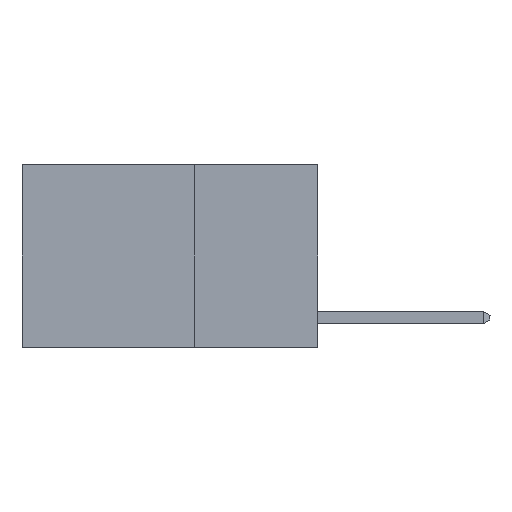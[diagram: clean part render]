
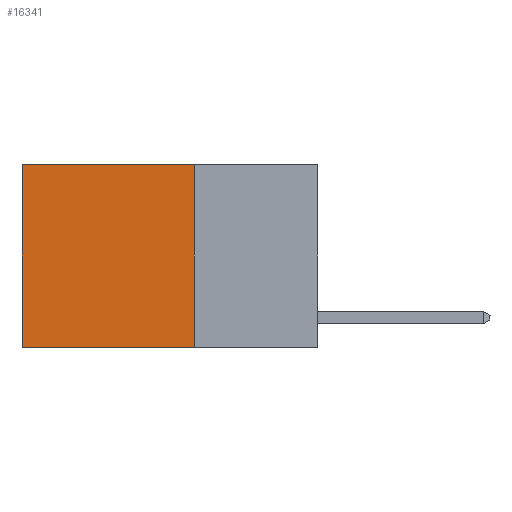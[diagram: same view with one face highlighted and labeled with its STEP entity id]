
A CAD part, left-side view. The second image highlights one B-rep face of the part: STEP entity #16341.
In plain terms, the highlighted planar face has unit normal (-1, 0, 0).
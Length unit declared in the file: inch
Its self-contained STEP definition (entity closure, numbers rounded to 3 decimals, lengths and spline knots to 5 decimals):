
#420 = CARTESIAN_POINT ( 'NONE',  ( 0.2625, 0.25, 0. ) ) ;
#433 = LINE ( 'NONE', #10669, #5865 ) ;
#895 = CARTESIAN_POINT ( 'NONE',  ( 0.2625, 0.25, 0. ) ) ;
#1762 = PLANE ( 'NONE',  #6375 ) ;
#1812 = ORIENTED_EDGE ( 'NONE', *, *, #13394, .F. ) ;
#3799 = EDGE_CURVE ( 'NONE', #4069, #9972, #10710, .T. ) ;
#4069 = VERTEX_POINT ( 'NONE', #8999 ) ;
#4175 = VERTEX_POINT ( 'NONE', #895 ) ;
#4338 = FACE_OUTER_BOUND ( 'NONE', #16299, .T. ) ;
#4739 = DIRECTION ( 'NONE',  ( 0., 1., 0. ) ) ;
#5096 = DIRECTION ( 'NONE',  ( 0., 0., -1. ) ) ;
#5238 = DIRECTION ( 'NONE',  ( 0., 0., -1. ) ) ;
#5668 = VECTOR ( 'NONE', #5238, 39.37008 ) ;
#5865 = VECTOR ( 'NONE', #5096, 39.37008 ) ;
#6375 = AXIS2_PLACEMENT_3D ( 'NONE', #420, #12952, #7456 ) ;
#7456 = DIRECTION ( 'NONE',  ( 0., 0., -1. ) ) ;
#8883 = CARTESIAN_POINT ( 'NONE',  ( 0.2625, 0.6, -0.37 ) ) ;
#8999 = CARTESIAN_POINT ( 'NONE',  ( 0.2625, 0.6, 0. ) ) ;
#9010 = CARTESIAN_POINT ( 'NONE',  ( 0.2625, 0.25, -0.37 ) ) ;
#9330 = LINE ( 'NONE', #15274, #12455 ) ;
#9401 = CARTESIAN_POINT ( 'NONE',  ( 0.2625, 0.25, -0.37 ) ) ;
#9972 = VERTEX_POINT ( 'NONE', #8883 ) ;
#10669 = CARTESIAN_POINT ( 'NONE',  ( 0.2625, 0.25, 0. ) ) ;
#10710 = LINE ( 'NONE', #10927, #5668 ) ;
#10927 = CARTESIAN_POINT ( 'NONE',  ( 0.2625, 0.6, 0. ) ) ;
#11186 = ORIENTED_EDGE ( 'NONE', *, *, #3799, .T. ) ;
#11480 = ORIENTED_EDGE ( 'NONE', *, *, #14968, .F. ) ;
#12455 = VECTOR ( 'NONE', #15452, 39.37008 ) ;
#12503 = VECTOR ( 'NONE', #4739, 39.37008 ) ;
#12833 = VERTEX_POINT ( 'NONE', #9401 ) ;
#12952 = DIRECTION ( 'NONE',  ( 1., 0., 0. ) ) ;
#13394 = EDGE_CURVE ( 'NONE', #4175, #12833, #433, .T. ) ;
#14114 = EDGE_CURVE ( 'NONE', #4175, #4069, #9330, .T. ) ;
#14968 = EDGE_CURVE ( 'NONE', #12833, #9972, #17688, .T. ) ;
#15274 = CARTESIAN_POINT ( 'NONE',  ( 0.2625, 0.25, 0. ) ) ;
#15452 = DIRECTION ( 'NONE',  ( 0., 1., 0. ) ) ;
#16299 = EDGE_LOOP ( 'NONE', ( #11186, #11480, #1812, #16791 ) ) ;
#16341 = ADVANCED_FACE ( 'NONE', ( #4338 ), #1762, .F. ) ;
#16791 = ORIENTED_EDGE ( 'NONE', *, *, #14114, .T. ) ;
#17688 = LINE ( 'NONE', #9010, #12503 ) ;
